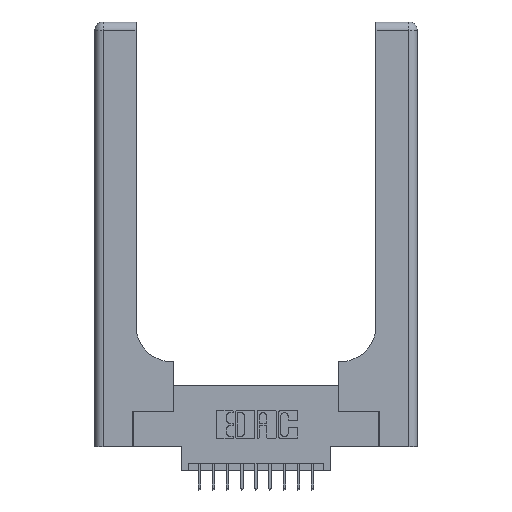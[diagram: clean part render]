
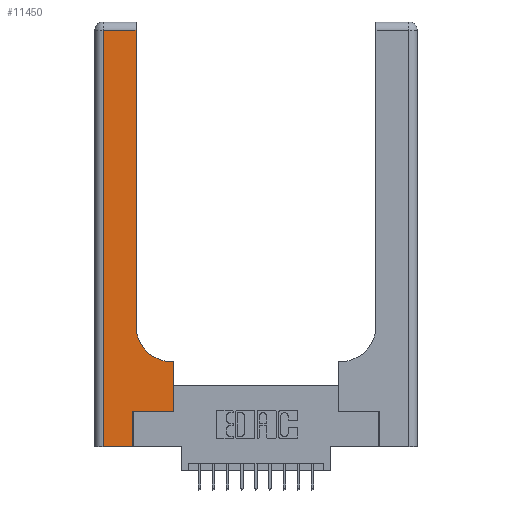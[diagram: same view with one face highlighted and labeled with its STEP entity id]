
A CAD part, top view. The second image highlights one B-rep face of the part: STEP entity #11450.
In plain terms, the highlighted planar face has unit normal (0, 0, 1).
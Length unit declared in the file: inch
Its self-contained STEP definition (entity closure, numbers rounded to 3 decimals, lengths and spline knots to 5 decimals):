
#18 = CARTESIAN_POINT ( 'NONE',  ( 0.2915, 3., 0.37 ) ) ;
#387 = VECTOR ( 'NONE', #10601, 39.37008 ) ;
#664 = VECTOR ( 'NONE', #13435, 39.37008 ) ;
#855 = CARTESIAN_POINT ( 'NONE',  ( 0.06, 0., 0.37 ) ) ;
#898 = LINE ( 'NONE', #6919, #664 ) ;
#1050 = EDGE_CURVE ( 'NONE', #5517, #9076, #1116, .T. ) ;
#1116 = LINE ( 'NONE', #18, #6341 ) ;
#1395 = DIRECTION ( 'NONE',  ( 0., 1., 0. ) ) ;
#2009 = CARTESIAN_POINT ( 'NONE',  ( 0.06, 3., 0.37 ) ) ;
#2675 = LINE ( 'NONE', #7951, #15432 ) ;
#3033 = LINE ( 'NONE', #5950, #11228 ) ;
#3228 = EDGE_LOOP ( 'NONE', ( #16264, #8061, #13853, #11660, #8006, #14054, #4432, #10455, #7009 ) ) ;
#3801 = VERTEX_POINT ( 'NONE', #9188 ) ;
#3956 = DIRECTION ( 'NONE',  ( 1., 0., 0. ) ) ;
#4039 = LINE ( 'NONE', #16206, #15375 ) ;
#4188 = DIRECTION ( 'NONE',  ( 1., 0., 0. ) ) ;
#4366 = EDGE_CURVE ( 'NONE', #6555, #10969, #12395, .T. ) ;
#4395 = DIRECTION ( 'NONE',  ( 0., 1., 0. ) ) ;
#4432 = ORIENTED_EDGE ( 'NONE', *, *, #8692, .T. ) ;
#4595 = FACE_OUTER_BOUND ( 'NONE', #3228, .T. ) ;
#5069 = DIRECTION ( 'NONE',  ( 0., 0., -1. ) ) ;
#5218 = CARTESIAN_POINT ( 'NONE',  ( 0.06, 2.94, 0.37 ) ) ;
#5460 = VERTEX_POINT ( 'NONE', #10560 ) ;
#5463 = AXIS2_PLACEMENT_3D ( 'NONE', #15043, #9879, #7310 ) ;
#5517 = VERTEX_POINT ( 'NONE', #15022 ) ;
#5603 = VECTOR ( 'NONE', #7274, 39.37008 ) ;
#5885 = VECTOR ( 'NONE', #4188, 39.37008 ) ;
#5950 = CARTESIAN_POINT ( 'NONE',  ( 0.269, 0., 0.37 ) ) ;
#6341 = VECTOR ( 'NONE', #15752, 39.37008 ) ;
#6555 = VERTEX_POINT ( 'NONE', #5218 ) ;
#6558 = EDGE_CURVE ( 'NONE', #5460, #3801, #10343, .T. ) ;
#6919 = CARTESIAN_POINT ( 'NONE',  ( 0., 2.94, 0.37 ) ) ;
#7009 = ORIENTED_EDGE ( 'NONE', *, *, #7662, .T. ) ;
#7144 = LINE ( 'NONE', #14973, #5885 ) ;
#7208 = CARTESIAN_POINT ( 'NONE',  ( 0.5585, 0.25, 0.37 ) ) ;
#7274 = DIRECTION ( 'NONE',  ( 0., -1., 0. ) ) ;
#7310 = DIRECTION ( 'NONE',  ( -1., 0., 0. ) ) ;
#7542 = CIRCLE ( 'NONE', #15409, 0.25 ) ;
#7662 = EDGE_CURVE ( 'NONE', #3801, #5517, #7542, .T. ) ;
#7951 = CARTESIAN_POINT ( 'NONE',  ( 0.5585, 0.25, 0.37 ) ) ;
#8006 = ORIENTED_EDGE ( 'NONE', *, *, #12266, .T. ) ;
#8061 = ORIENTED_EDGE ( 'NONE', *, *, #14386, .T. ) ;
#8591 = PLANE ( 'NONE',  #5463 ) ;
#8692 = EDGE_CURVE ( 'NONE', #9461, #5460, #2675, .T. ) ;
#8956 = EDGE_CURVE ( 'NONE', #13619, #9461, #7144, .T. ) ;
#9076 = VERTEX_POINT ( 'NONE', #9362 ) ;
#9188 = CARTESIAN_POINT ( 'NONE',  ( 0.5415, 0.6, 0.37 ) ) ;
#9362 = CARTESIAN_POINT ( 'NONE',  ( 0.2915, 2.94, 0.37 ) ) ;
#9461 = VERTEX_POINT ( 'NONE', #7208 ) ;
#9569 = DIRECTION ( 'NONE',  ( 1., 0., 0. ) ) ;
#9879 = DIRECTION ( 'NONE',  ( 0., 0., -1. ) ) ;
#10343 = LINE ( 'NONE', #15668, #387 ) ;
#10455 = ORIENTED_EDGE ( 'NONE', *, *, #6558, .T. ) ;
#10560 = CARTESIAN_POINT ( 'NONE',  ( 0.5585, 0.6, 0.37 ) ) ;
#10601 = DIRECTION ( 'NONE',  ( -1., 0., 0. ) ) ;
#10969 = VERTEX_POINT ( 'NONE', #855 ) ;
#11228 = VECTOR ( 'NONE', #4395, 39.37008 ) ;
#11450 = ADVANCED_FACE ( 'NONE', ( #4595 ), #8591, .F. ) ;
#11479 = CARTESIAN_POINT ( 'NONE',  ( 0.269, 0., 0.37 ) ) ;
#11660 = ORIENTED_EDGE ( 'NONE', *, *, #15333, .T. ) ;
#12266 = EDGE_CURVE ( 'NONE', #16110, #13619, #3033, .T. ) ;
#12395 = LINE ( 'NONE', #2009, #5603 ) ;
#13435 = DIRECTION ( 'NONE',  ( -1., 0., 0. ) ) ;
#13619 = VERTEX_POINT ( 'NONE', #16100 ) ;
#13853 = ORIENTED_EDGE ( 'NONE', *, *, #4366, .T. ) ;
#14054 = ORIENTED_EDGE ( 'NONE', *, *, #8956, .T. ) ;
#14386 = EDGE_CURVE ( 'NONE', #9076, #6555, #898, .T. ) ;
#14973 = CARTESIAN_POINT ( 'NONE',  ( 0.269, 0.25, 0.37 ) ) ;
#15022 = CARTESIAN_POINT ( 'NONE',  ( 0.2915, 0.85, 0.37 ) ) ;
#15043 = CARTESIAN_POINT ( 'NONE',  ( 0., 3., 0.37 ) ) ;
#15333 = EDGE_CURVE ( 'NONE', #10969, #16110, #4039, .T. ) ;
#15375 = VECTOR ( 'NONE', #9569, 39.37008 ) ;
#15409 = AXIS2_PLACEMENT_3D ( 'NONE', #15687, #5069, #3956 ) ;
#15432 = VECTOR ( 'NONE', #1395, 39.37008 ) ;
#15668 = CARTESIAN_POINT ( 'NONE',  ( 0.2915, 0.6, 0.37 ) ) ;
#15687 = CARTESIAN_POINT ( 'NONE',  ( 0.5415, 0.85, 0.37 ) ) ;
#15752 = DIRECTION ( 'NONE',  ( 0., 1., 0. ) ) ;
#16100 = CARTESIAN_POINT ( 'NONE',  ( 0.269, 0.25, 0.37 ) ) ;
#16110 = VERTEX_POINT ( 'NONE', #11479 ) ;
#16206 = CARTESIAN_POINT ( 'NONE',  ( 0., 0., 0.37 ) ) ;
#16264 = ORIENTED_EDGE ( 'NONE', *, *, #1050, .T. ) ;
